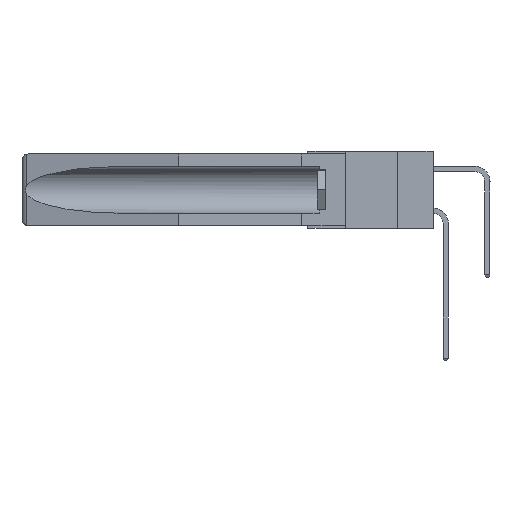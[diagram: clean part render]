
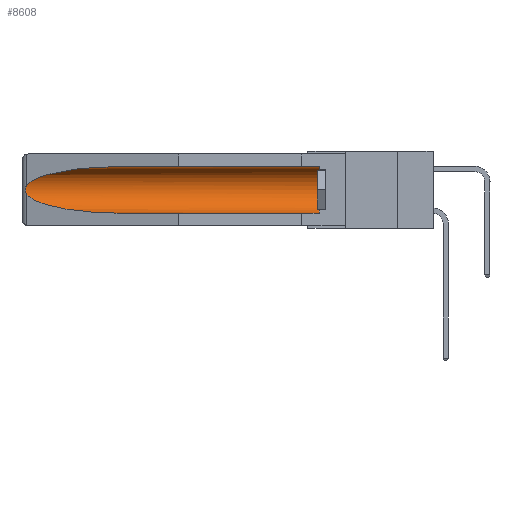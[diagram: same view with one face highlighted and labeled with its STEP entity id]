
A CAD part, left-side view. The second image highlights one B-rep face of the part: STEP entity #8608.
In plain terms, the highlighted cylindrical face has radius 2.857 mm (diameter 5.715 mm), a partial arc.
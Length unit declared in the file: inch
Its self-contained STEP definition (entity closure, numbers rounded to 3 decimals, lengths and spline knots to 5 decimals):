
#313 = CARTESIAN_POINT ( 'NONE',  ( 0.2673, 1.5327, -0.16383 ) ) ;
#395 = CARTESIAN_POINT ( 'NONE',  ( 0.155, 1.07973, -0.284 ) ) ;
#540 = CARTESIAN_POINT ( 'NONE',  ( 0.155, 0.126, -0.284 ) ) ;
#1012 = CARTESIAN_POINT ( 'NONE',  ( 0.155, 0.126, -0.059 ) ) ;
#1236 = CARTESIAN_POINT ( 'NONE',  ( 0.21114, 1.30732, -0.284 ) ) ;
#1274 = VECTOR ( 'NONE', #26639, 39.37008 ) ;
#2028 = CARTESIAN_POINT ( 'NONE',  ( 0.26654, 1.53092, -0.15636 ) ) ;
#2530 = CARTESIAN_POINT ( 'NONE',  ( 0.2675, 1.53308, -0.17534 ) ) ;
#3240 = CARTESIAN_POINT ( 'NONE',  ( 0.155, -0.30754, -0.1715 ) ) ;
#4229 = CARTESIAN_POINT ( 'NONE',  ( 0.2675, 1.53308, -0.16763 ) ) ;
#4588 = CARTESIAN_POINT ( 'NONE',  ( 0.26537, 1.52718, -0.19328 ) ) ;
#5230 = EDGE_LOOP ( 'NONE', ( #17476, #23866, #19927, #16083, #8849, #20733 ) ) ;
#6032 = DIRECTION ( 'NONE',  ( 0., -1., 0. ) ) ;
#7260 = VERTEX_POINT ( 'NONE', #1012 ) ;
#8608 = ADVANCED_FACE ( 'NONE', ( #29321 ), #28930, .F. ) ;
#8747 =( BOUNDED_CURVE ( )  B_SPLINE_CURVE ( 3, ( #24651, #20244, #15729, #22647 ),
 .UNSPECIFIED., .F., .F. ) 
 B_SPLINE_CURVE_WITH_KNOTS ( ( 4, 4 ),
 ( 4.71239, 6.08839 ),
 .UNSPECIFIED. ) 
 CURVE ( )  GEOMETRIC_REPRESENTATION_ITEM ( )  RATIONAL_B_SPLINE_CURVE ( ( 1., 0.848, 0.848, 1. ) ) 
 REPRESENTATION_ITEM ( '' )  );
#8849 = ORIENTED_EDGE ( 'NONE', *, *, #24799, .T. ) ;
#8992 = CARTESIAN_POINT ( 'NONE',  ( 0.155, -0.30754, -0.284 ) ) ;
#9222 = VERTEX_POINT ( 'NONE', #395 ) ;
#9460 = CARTESIAN_POINT ( 'NONE',  ( 0.26597, 1.52961, -0.15275 ) ) ;
#10979 = B_SPLINE_CURVE_WITH_KNOTS ( 'NONE', 3,
 ( #14014, #9460, #2028, #313, #4229, #2530, #18820, #15824, #29610, #18136 ),
 .UNSPECIFIED., .F., .F.,
 ( 4, 2, 2, 2, 4 ),
 ( 0., 0.00029, 0.00058, 0.00087, 0.00117 ),
 .UNSPECIFIED. ) ;
#11593 = CARTESIAN_POINT ( 'NONE',  ( 0.26537, 1.52718, -0.19328 ) ) ;
#11711 = VERTEX_POINT ( 'NONE', #18167 ) ;
#11800 = VERTEX_POINT ( 'NONE', #11593 ) ;
#12822 = CARTESIAN_POINT ( 'NONE',  ( 0.155, 0.126, -0.1715 ) ) ;
#13129 = CARTESIAN_POINT ( 'NONE',  ( 0.26537, 1.52718, -0.14972 ) ) ;
#14014 = CARTESIAN_POINT ( 'NONE',  ( 0.26537, 1.52718, -0.14972 ) ) ;
#14037 = AXIS2_PLACEMENT_3D ( 'NONE', #3240, #28510, #14664 ) ;
#14664 = DIRECTION ( 'NONE',  ( 0., 0., 1. ) ) ;
#15729 = CARTESIAN_POINT ( 'NONE',  ( 0.25451, 1.48313, -0.09465 ) ) ;
#15824 = CARTESIAN_POINT ( 'NONE',  ( 0.26655, 1.53094, -0.18657 ) ) ;
#16083 = ORIENTED_EDGE ( 'NONE', *, *, #25518, .F. ) ;
#16190 = EDGE_CURVE ( 'NONE', #27524, #11800, #10979, .T. ) ;
#17476 = ORIENTED_EDGE ( 'NONE', *, *, #22820, .T. ) ;
#18019 = EDGE_CURVE ( 'NONE', #11800, #9222, #26116, .T. ) ;
#18136 = CARTESIAN_POINT ( 'NONE',  ( 0.26537, 1.52718, -0.19328 ) ) ;
#18167 = CARTESIAN_POINT ( 'NONE',  ( 0.155, 1.07973, -0.059 ) ) ;
#18820 = CARTESIAN_POINT ( 'NONE',  ( 0.2673, 1.53269, -0.17917 ) ) ;
#19444 = VERTEX_POINT ( 'NONE', #540 ) ;
#19927 = ORIENTED_EDGE ( 'NONE', *, *, #18019, .T. ) ;
#20244 = CARTESIAN_POINT ( 'NONE',  ( 0.21114, 1.30732, -0.059 ) ) ;
#20733 = ORIENTED_EDGE ( 'NONE', *, *, #27535, .T. ) ;
#22647 = CARTESIAN_POINT ( 'NONE',  ( 0.26537, 1.52718, -0.14972 ) ) ;
#22820 = EDGE_CURVE ( 'NONE', #11711, #27524, #8747, .T. ) ;
#23726 = CIRCLE ( 'NONE', #28169, 0.1125 ) ;
#23866 = ORIENTED_EDGE ( 'NONE', *, *, #16190, .T. ) ;
#24651 = CARTESIAN_POINT ( 'NONE',  ( 0.155, 1.07973, -0.059 ) ) ;
#24799 = EDGE_CURVE ( 'NONE', #19444, #7260, #23726, .T. ) ;
#24804 = VECTOR ( 'NONE', #27229, 39.37008 ) ;
#25518 = EDGE_CURVE ( 'NONE', #19444, #9222, #28788, .T. ) ;
#26116 =( BOUNDED_CURVE ( )  B_SPLINE_CURVE ( 3, ( #4588, #27832, #1236, #28801 ),
 .UNSPECIFIED., .F., .F. ) 
 B_SPLINE_CURVE_WITH_KNOTS ( ( 4, 4 ),
 ( 0.1948, 1.5708 ),
 .UNSPECIFIED. ) 
 CURVE ( )  GEOMETRIC_REPRESENTATION_ITEM ( )  RATIONAL_B_SPLINE_CURVE ( ( 1., 0.848, 0.848, 1. ) ) 
 REPRESENTATION_ITEM ( '' )  );
#26639 = DIRECTION ( 'NONE',  ( 0., 1., 0. ) ) ;
#27029 = DIRECTION ( 'NONE',  ( 0., 0., 1. ) ) ;
#27203 = LINE ( 'NONE', #29241, #1274 ) ;
#27229 = DIRECTION ( 'NONE',  ( 0., 1., 0. ) ) ;
#27524 = VERTEX_POINT ( 'NONE', #13129 ) ;
#27535 = EDGE_CURVE ( 'NONE', #7260, #11711, #27203, .T. ) ;
#27832 = CARTESIAN_POINT ( 'NONE',  ( 0.25451, 1.48313, -0.24835 ) ) ;
#28169 = AXIS2_PLACEMENT_3D ( 'NONE', #12822, #6032, #27029 ) ;
#28510 = DIRECTION ( 'NONE',  ( 0., 1., 0. ) ) ;
#28788 = LINE ( 'NONE', #8992, #24804 ) ;
#28801 = CARTESIAN_POINT ( 'NONE',  ( 0.155, 1.07973, -0.284 ) ) ;
#28930 = CYLINDRICAL_SURFACE ( 'NONE', #14037, 0.1125 ) ;
#29241 = CARTESIAN_POINT ( 'NONE',  ( 0.155, -0.30754, -0.059 ) ) ;
#29321 = FACE_OUTER_BOUND ( 'NONE', #5230, .T. ) ;
#29610 = CARTESIAN_POINT ( 'NONE',  ( 0.26597, 1.5296, -0.19026 ) ) ;
